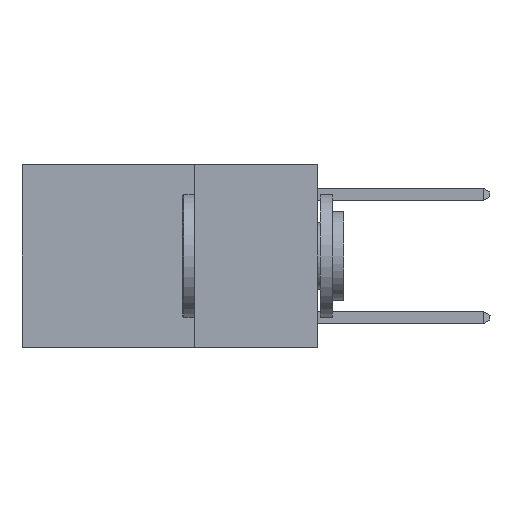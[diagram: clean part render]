
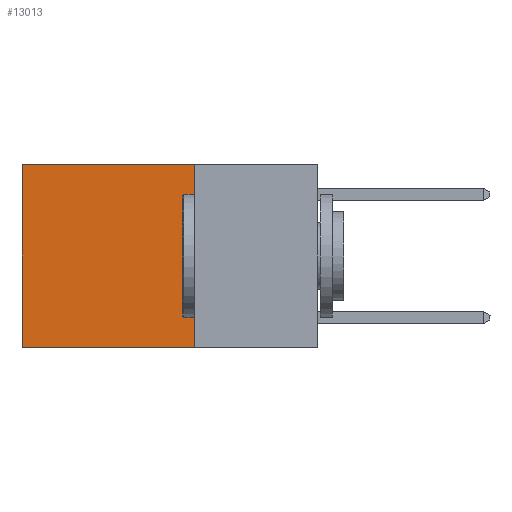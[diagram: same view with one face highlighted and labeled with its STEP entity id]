
A CAD part, left-side view. The second image highlights one B-rep face of the part: STEP entity #13013.
In plain terms, the highlighted planar face has unit normal (-1, 0, 0).
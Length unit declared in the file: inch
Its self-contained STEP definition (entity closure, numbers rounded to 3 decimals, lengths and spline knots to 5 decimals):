
#1 = CARTESIAN_POINT ( 'NONE',  ( 0.2625, 0.25, 0. ) ) ;
#549 = CARTESIAN_POINT ( 'NONE',  ( 0.2625, 0.25, 0. ) ) ;
#2349 = VERTEX_POINT ( 'NONE', #15381 ) ;
#4494 = LINE ( 'NONE', #1, #19776 ) ;
#5055 = DIRECTION ( 'NONE',  ( 0., 0., -1. ) ) ;
#5670 = ORIENTED_EDGE ( 'NONE', *, *, #5883, .F. ) ;
#5838 = PLANE ( 'NONE',  #22910 ) ;
#5848 = VERTEX_POINT ( 'NONE', #15393 ) ;
#5883 = EDGE_CURVE ( 'NONE', #2349, #6816, #9473, .T. ) ;
#6816 = VERTEX_POINT ( 'NONE', #16643 ) ;
#8491 = ORIENTED_EDGE ( 'NONE', *, *, #21376, .T. ) ;
#9473 = LINE ( 'NONE', #27965, #21218 ) ;
#10579 = EDGE_CURVE ( 'NONE', #5848, #12797, #4494, .T. ) ;
#11377 = LINE ( 'NONE', #31096, #23872 ) ;
#12797 = VERTEX_POINT ( 'NONE', #15225 ) ;
#13012 = FACE_OUTER_BOUND ( 'NONE', #27525, .T. ) ;
#13013 = ADVANCED_FACE ( 'NONE', ( #13012 ), #5838, .F. ) ;
#13814 = DIRECTION ( 'NONE',  ( 1., 0., 0. ) ) ;
#15225 = CARTESIAN_POINT ( 'NONE',  ( 0.2625, 0.6, 0. ) ) ;
#15381 = CARTESIAN_POINT ( 'NONE',  ( 0.2625, 0.25, -0.37 ) ) ;
#15393 = CARTESIAN_POINT ( 'NONE',  ( 0.2625, 0.25, 0. ) ) ;
#16480 = DIRECTION ( 'NONE',  ( 0., 0., -1. ) ) ;
#16643 = CARTESIAN_POINT ( 'NONE',  ( 0.2625, 0.6, -0.37 ) ) ;
#19776 = VECTOR ( 'NONE', #27168, 39.37008 ) ;
#21218 = VECTOR ( 'NONE', #25547, 39.37008 ) ;
#21376 = EDGE_CURVE ( 'NONE', #12797, #6816, #11377, .T. ) ;
#22910 = AXIS2_PLACEMENT_3D ( 'NONE', #23457, #13814, #30327 ) ;
#23457 = CARTESIAN_POINT ( 'NONE',  ( 0.2625, 0.25, 0. ) ) ;
#23553 = ORIENTED_EDGE ( 'NONE', *, *, #10579, .T. ) ;
#23872 = VECTOR ( 'NONE', #16480, 39.37008 ) ;
#25547 = DIRECTION ( 'NONE',  ( 0., 1., 0. ) ) ;
#26761 = VECTOR ( 'NONE', #5055, 39.37008 ) ;
#27168 = DIRECTION ( 'NONE',  ( 0., 1., 0. ) ) ;
#27503 = ORIENTED_EDGE ( 'NONE', *, *, #31668, .F. ) ;
#27525 = EDGE_LOOP ( 'NONE', ( #8491, #5670, #27503, #23553 ) ) ;
#27965 = CARTESIAN_POINT ( 'NONE',  ( 0.2625, 0.25, -0.37 ) ) ;
#29096 = LINE ( 'NONE', #549, #26761 ) ;
#30327 = DIRECTION ( 'NONE',  ( 0., 0., -1. ) ) ;
#31096 = CARTESIAN_POINT ( 'NONE',  ( 0.2625, 0.6, 0. ) ) ;
#31668 = EDGE_CURVE ( 'NONE', #5848, #2349, #29096, .T. ) ;
